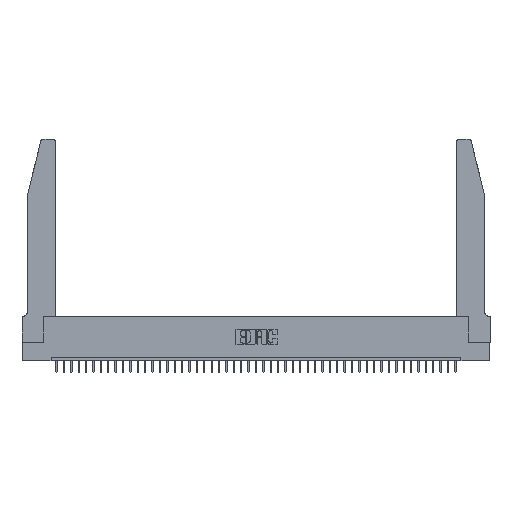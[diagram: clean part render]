
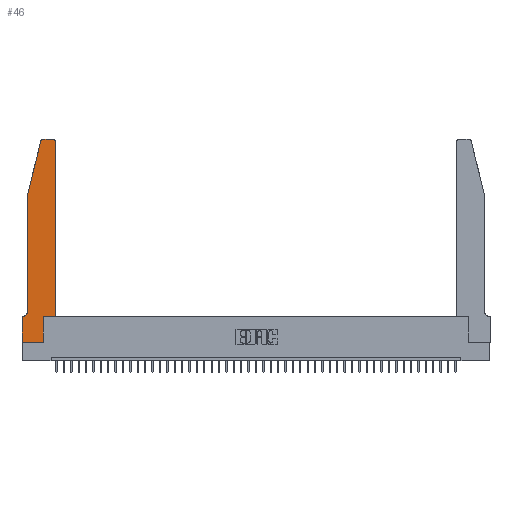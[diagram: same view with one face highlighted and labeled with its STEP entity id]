
A CAD part, top view. The second image highlights one B-rep face of the part: STEP entity #46.
In plain terms, the highlighted planar face has unit normal (0, 0, 1).
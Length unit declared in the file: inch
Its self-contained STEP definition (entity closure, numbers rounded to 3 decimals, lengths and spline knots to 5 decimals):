
#46 = ADVANCED_FACE ( 'NONE', ( #29631 ), #40268, .T. ) ;
#299 = CIRCLE ( 'NONE', #22207, 0.07 ) ;
#493 = VECTOR ( 'NONE', #24073, 39.37008 ) ;
#1655 = CARTESIAN_POINT ( 'NONE',  ( 0.4505, 0.35, 0.37 ) ) ;
#1718 = ORIENTED_EDGE ( 'NONE', *, *, #5313, .T. ) ;
#2055 = ORIENTED_EDGE ( 'NONE', *, *, #17649, .T. ) ;
#3326 = VERTEX_POINT ( 'NONE', #17317 ) ;
#3441 = ORIENTED_EDGE ( 'NONE', *, *, #32471, .T. ) ;
#3476 = CARTESIAN_POINT ( 'NONE',  ( 0.4505, 0.35, 0.37 ) ) ;
#3501 = EDGE_CURVE ( 'NONE', #21246, #26945, #24310, .T. ) ;
#3666 = DIRECTION ( 'NONE',  ( 0., 0., 1. ) ) ;
#3809 = DIRECTION ( 'NONE',  ( 0., -1., 0. ) ) ;
#4387 = VERTEX_POINT ( 'NONE', #16786 ) ;
#5313 = EDGE_CURVE ( 'NONE', #36850, #22278, #24162, .T. ) ;
#5672 = DIRECTION ( 'NONE',  ( 0., 0., -1. ) ) ;
#5726 = VECTOR ( 'NONE', #35516, 39.37008 ) ;
#8834 = VERTEX_POINT ( 'NONE', #36697 ) ;
#8891 = ORIENTED_EDGE ( 'NONE', *, *, #20327, .T. ) ;
#9801 = ORIENTED_EDGE ( 'NONE', *, *, #41186, .T. ) ;
#10585 = CARTESIAN_POINT ( 'NONE',  ( 0.4205, 2.72, 0.37 ) ) ;
#10868 = DIRECTION ( 'NONE',  ( 1., 0., 0. ) ) ;
#12659 = CARTESIAN_POINT ( 'NONE',  ( 0., 0.35, 0.37 ) ) ;
#13436 = CIRCLE ( 'NONE', #20432, 0.03 ) ;
#14347 = EDGE_CURVE ( 'NONE', #3326, #8834, #33659, .T. ) ;
#15190 = CARTESIAN_POINT ( 'NONE',  ( 0.0755, 0.35, 0.37 ) ) ;
#15522 = CARTESIAN_POINT ( 'NONE',  ( 0.2865, 0., 0.37 ) ) ;
#16118 = CARTESIAN_POINT ( 'NONE',  ( 0.2865, 0.35, 0.37 ) ) ;
#16145 = CARTESIAN_POINT ( 'NONE',  ( 0.284, 2.72, 0.37 ) ) ;
#16786 = CARTESIAN_POINT ( 'NONE',  ( 0.0755, 0.42, 0.37 ) ) ;
#17144 = DIRECTION ( 'NONE',  ( 1., 0., 0. ) ) ;
#17317 = CARTESIAN_POINT ( 'NONE',  ( 0.4205, 2.75, 0.37 ) ) ;
#17492 = LINE ( 'NONE', #35507, #23962 ) ;
#17649 = EDGE_CURVE ( 'NONE', #41140, #17837, #25809, .T. ) ;
#17837 = VERTEX_POINT ( 'NONE', #29334 ) ;
#17926 = DIRECTION ( 'NONE',  ( 0., 1., 0. ) ) ;
#18049 = DIRECTION ( 'NONE',  ( -0.239, -0.971, 0. ) ) ;
#18544 = LINE ( 'NONE', #3476, #37470 ) ;
#18744 = EDGE_LOOP ( 'NONE', ( #36581, #25722, #2055, #34655, #33558, #3441, #9801, #26933, #8891, #1718, #27036, #40806 ) ) ;
#18820 = EDGE_CURVE ( 'NONE', #8834, #41140, #13436, .T. ) ;
#19537 = EDGE_CURVE ( 'NONE', #37200, #3326, #31575, .T. ) ;
#20226 = EDGE_CURVE ( 'NONE', #22278, #37200, #18544, .T. ) ;
#20327 = EDGE_CURVE ( 'NONE', #26945, #36850, #17492, .T. ) ;
#20432 = AXIS2_PLACEMENT_3D ( 'NONE', #16145, #43616, #29978 ) ;
#20639 = CARTESIAN_POINT ( 'NONE',  ( 0.25487, 2.72718, 0.37 ) ) ;
#20723 = AXIS2_PLACEMENT_3D ( 'NONE', #10585, #3666, #10868 ) ;
#21246 = VERTEX_POINT ( 'NONE', #21959 ) ;
#21959 = CARTESIAN_POINT ( 'NONE',  ( 0., 0., 0.37 ) ) ;
#22124 = CARTESIAN_POINT ( 'NONE',  ( 0.0755, 2., 0.37 ) ) ;
#22207 = AXIS2_PLACEMENT_3D ( 'NONE', #35102, #5672, #35477 ) ;
#22278 = VERTEX_POINT ( 'NONE', #23684 ) ;
#22655 = DIRECTION ( 'NONE',  ( 1., 0., 0. ) ) ;
#23262 = VECTOR ( 'NONE', #17144, 39.37008 ) ;
#23684 = CARTESIAN_POINT ( 'NONE',  ( 0.4505, 0.35, 0.37 ) ) ;
#23958 = CARTESIAN_POINT ( 'NONE',  ( 0.0755, 2., 0.37 ) ) ;
#23962 = VECTOR ( 'NONE', #17926, 39.37008 ) ;
#23974 = LINE ( 'NONE', #22124, #5726 ) ;
#24073 = DIRECTION ( 'NONE',  ( 1., 0., 0. ) ) ;
#24162 = LINE ( 'NONE', #1655, #493 ) ;
#24310 = LINE ( 'NONE', #34255, #23262 ) ;
#25169 = DIRECTION ( 'NONE',  ( 0., 1., 0. ) ) ;
#25722 = ORIENTED_EDGE ( 'NONE', *, *, #18820, .T. ) ;
#25809 = LINE ( 'NONE', #23958, #38182 ) ;
#26933 = ORIENTED_EDGE ( 'NONE', *, *, #3501, .T. ) ;
#26945 = VERTEX_POINT ( 'NONE', #15522 ) ;
#27036 = ORIENTED_EDGE ( 'NONE', *, *, #20226, .T. ) ;
#27242 = VECTOR ( 'NONE', #3809, 39.37008 ) ;
#28566 = VECTOR ( 'NONE', #42238, 39.37008 ) ;
#29152 = CARTESIAN_POINT ( 'NONE',  ( 0.0055, 0.35, 0.37 ) ) ;
#29334 = CARTESIAN_POINT ( 'NONE',  ( 0.0755, 2., 0.37 ) ) ;
#29631 = FACE_OUTER_BOUND ( 'NONE', #18744, .T. ) ;
#29978 = DIRECTION ( 'NONE',  ( 1., 0., 0. ) ) ;
#31575 = CIRCLE ( 'NONE', #20723, 0.03 ) ;
#32471 = EDGE_CURVE ( 'NONE', #40022, #43861, #37764, .T. ) ;
#32596 = VECTOR ( 'NONE', #40054, 39.37008 ) ;
#32598 = LINE ( 'NONE', #37792, #27242 ) ;
#32947 = CARTESIAN_POINT ( 'NONE',  ( 0., 0.35, 0.37 ) ) ;
#33558 = ORIENTED_EDGE ( 'NONE', *, *, #33964, .T. ) ;
#33659 = LINE ( 'NONE', #39902, #32596 ) ;
#33964 = EDGE_CURVE ( 'NONE', #4387, #40022, #299, .T. ) ;
#34255 = CARTESIAN_POINT ( 'NONE',  ( 0., 0., 0.37 ) ) ;
#34655 = ORIENTED_EDGE ( 'NONE', *, *, #40989, .T. ) ;
#35102 = CARTESIAN_POINT ( 'NONE',  ( 0.0055, 0.42, 0.37 ) ) ;
#35477 = DIRECTION ( 'NONE',  ( -1., 0., 0. ) ) ;
#35507 = CARTESIAN_POINT ( 'NONE',  ( 0.2865, 0.35, 0.37 ) ) ;
#35516 = DIRECTION ( 'NONE',  ( 0., -1., 0. ) ) ;
#36581 = ORIENTED_EDGE ( 'NONE', *, *, #14347, .T. ) ;
#36650 = DIRECTION ( 'NONE',  ( 0., 0., 1. ) ) ;
#36697 = CARTESIAN_POINT ( 'NONE',  ( 0.284, 2.75, 0.37 ) ) ;
#36850 = VERTEX_POINT ( 'NONE', #16118 ) ;
#37200 = VERTEX_POINT ( 'NONE', #39810 ) ;
#37470 = VECTOR ( 'NONE', #25169, 39.37008 ) ;
#37764 = LINE ( 'NONE', #15190, #28566 ) ;
#37792 = CARTESIAN_POINT ( 'NONE',  ( 0., 0., 0.37 ) ) ;
#38182 = VECTOR ( 'NONE', #18049, 39.37008 ) ;
#38970 = AXIS2_PLACEMENT_3D ( 'NONE', #12659, #36650, #22655 ) ;
#39810 = CARTESIAN_POINT ( 'NONE',  ( 0.4505, 2.72, 0.37 ) ) ;
#39902 = CARTESIAN_POINT ( 'NONE',  ( 0.2605, 2.75, 0.37 ) ) ;
#40022 = VERTEX_POINT ( 'NONE', #29152 ) ;
#40054 = DIRECTION ( 'NONE',  ( -1., 0., 0. ) ) ;
#40268 = PLANE ( 'NONE',  #38970 ) ;
#40806 = ORIENTED_EDGE ( 'NONE', *, *, #19537, .T. ) ;
#40989 = EDGE_CURVE ( 'NONE', #17837, #4387, #23974, .T. ) ;
#41140 = VERTEX_POINT ( 'NONE', #20639 ) ;
#41186 = EDGE_CURVE ( 'NONE', #43861, #21246, #32598, .T. ) ;
#42238 = DIRECTION ( 'NONE',  ( -1., 0., 0. ) ) ;
#43616 = DIRECTION ( 'NONE',  ( 0., 0., 1. ) ) ;
#43861 = VERTEX_POINT ( 'NONE', #32947 ) ;
